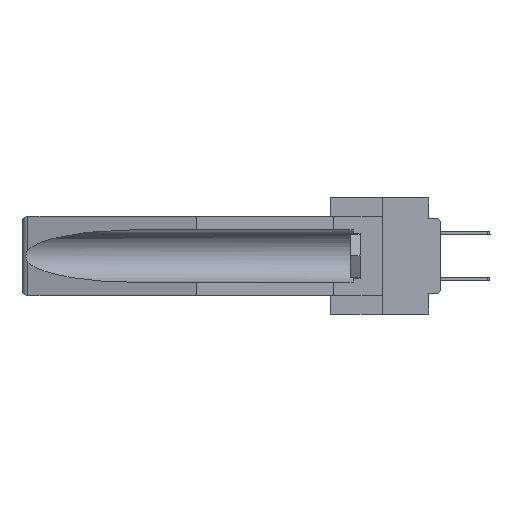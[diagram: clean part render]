
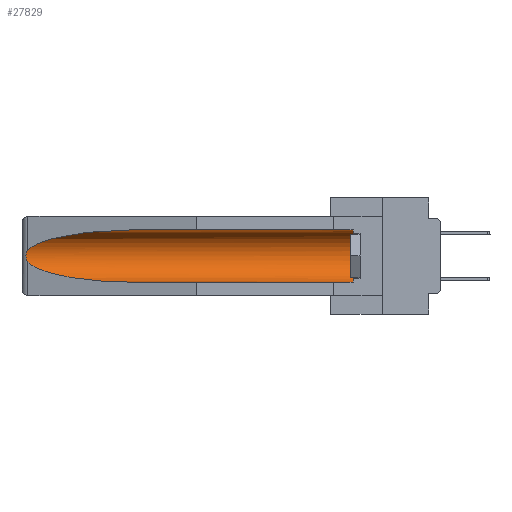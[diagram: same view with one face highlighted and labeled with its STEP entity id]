
A CAD part, left-side view. The second image highlights one B-rep face of the part: STEP entity #27829.
In plain terms, the highlighted cylindrical face has radius 2.857 mm (diameter 5.715 mm), a partial arc.
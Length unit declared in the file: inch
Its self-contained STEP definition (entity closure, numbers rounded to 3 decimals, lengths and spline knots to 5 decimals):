
#566 = VERTEX_POINT ( 'NONE', #17553 ) ;
#653 = CARTESIAN_POINT ( 'NONE',  ( 0.155, 1.07973, -0.059 ) ) ;
#687 = DIRECTION ( 'NONE',  ( 0., 1., 0. ) ) ;
#1659 = LINE ( 'NONE', #16210, #16730 ) ;
#2113 = DIRECTION ( 'NONE',  ( 0., 0., 1. ) ) ;
#2228 = VERTEX_POINT ( 'NONE', #9669 ) ;
#2504 = CARTESIAN_POINT ( 'NONE',  ( 0.155, -0.30754, -0.059 ) ) ;
#3400 = EDGE_LOOP ( 'NONE', ( #4878, #9230, #28040, #16546, #22907, #12775 ) ) ;
#3964 = CARTESIAN_POINT ( 'NONE',  ( 0.2673, 1.5327, -0.16383 ) ) ;
#4175 = CARTESIAN_POINT ( 'NONE',  ( 0.155, 0.126, -0.1715 ) ) ;
#4479 = CARTESIAN_POINT ( 'NONE',  ( 0.155, 1.07973, -0.284 ) ) ;
#4579 = AXIS2_PLACEMENT_3D ( 'NONE', #8742, #15077, #15179 ) ;
#4878 = ORIENTED_EDGE ( 'NONE', *, *, #25182, .T. ) ;
#4927 = FACE_OUTER_BOUND ( 'NONE', #3400, .T. ) ;
#5553 = EDGE_CURVE ( 'NONE', #22213, #27529, #18451, .T. ) ;
#5556 = VERTEX_POINT ( 'NONE', #4479 ) ;
#5742 = CARTESIAN_POINT ( 'NONE',  ( 0.26537, 1.52718, -0.14972 ) ) ;
#6900 = VECTOR ( 'NONE', #22388, 39.37008 ) ;
#7193 =( BOUNDED_CURVE ( )  B_SPLINE_CURVE ( 3, ( #27815, #12310, #20849, #20941 ),
 .UNSPECIFIED., .F., .F. ) 
 B_SPLINE_CURVE_WITH_KNOTS ( ( 4, 4 ),
 ( 0.1948, 1.5708 ),
 .UNSPECIFIED. ) 
 CURVE ( )  GEOMETRIC_REPRESENTATION_ITEM ( )  RATIONAL_B_SPLINE_CURVE ( ( 1., 0.848, 0.848, 1. ) ) 
 REPRESENTATION_ITEM ( '' )  );
#8714 = EDGE_CURVE ( 'NONE', #17061, #2228, #9009, .T. ) ;
#8742 = CARTESIAN_POINT ( 'NONE',  ( 0.155, -0.30754, -0.1715 ) ) ;
#9009 = B_SPLINE_CURVE_WITH_KNOTS ( 'NONE', 3,
 ( #14926, #10539, #17366, #3964, #24130, #10717, #12950, #22350, #15322, #17951 ),
 .UNSPECIFIED., .F., .F.,
 ( 4, 2, 2, 2, 4 ),
 ( 0., 0.00029, 0.00058, 0.00087, 0.00117 ),
 .UNSPECIFIED. ) ;
#9230 = ORIENTED_EDGE ( 'NONE', *, *, #8714, .T. ) ;
#9669 = CARTESIAN_POINT ( 'NONE',  ( 0.26537, 1.52718, -0.19328 ) ) ;
#10539 = CARTESIAN_POINT ( 'NONE',  ( 0.26597, 1.52961, -0.15275 ) ) ;
#10717 = CARTESIAN_POINT ( 'NONE',  ( 0.2675, 1.53308, -0.17534 ) ) ;
#11612 = CARTESIAN_POINT ( 'NONE',  ( 0.21114, 1.30732, -0.059 ) ) ;
#12089 = CARTESIAN_POINT ( 'NONE',  ( 0.25451, 1.48313, -0.09465 ) ) ;
#12310 = CARTESIAN_POINT ( 'NONE',  ( 0.25451, 1.48313, -0.24835 ) ) ;
#12775 = ORIENTED_EDGE ( 'NONE', *, *, #5553, .T. ) ;
#12950 = CARTESIAN_POINT ( 'NONE',  ( 0.2673, 1.53269, -0.17917 ) ) ;
#14926 = CARTESIAN_POINT ( 'NONE',  ( 0.26537, 1.52718, -0.14972 ) ) ;
#15077 = DIRECTION ( 'NONE',  ( 0., 1., 0. ) ) ;
#15137 = CIRCLE ( 'NONE', #19464, 0.1125 ) ;
#15179 = DIRECTION ( 'NONE',  ( 0., 0., 1. ) ) ;
#15322 = CARTESIAN_POINT ( 'NONE',  ( 0.26597, 1.5296, -0.19026 ) ) ;
#15541 = DIRECTION ( 'NONE',  ( 0., -1., 0. ) ) ;
#16210 = CARTESIAN_POINT ( 'NONE',  ( 0.155, -0.30754, -0.284 ) ) ;
#16346 =( BOUNDED_CURVE ( )  B_SPLINE_CURVE ( 3, ( #25039, #11612, #12089, #21002 ),
 .UNSPECIFIED., .F., .T. ) 
 B_SPLINE_CURVE_WITH_KNOTS ( ( 4, 4 ),
 ( 4.71239, 6.08839 ),
 .UNSPECIFIED. ) 
 CURVE ( )  GEOMETRIC_REPRESENTATION_ITEM ( )  RATIONAL_B_SPLINE_CURVE ( ( 1., 0.848, 0.848, 1. ) ) 
 REPRESENTATION_ITEM ( '' )  );
#16498 = CARTESIAN_POINT ( 'NONE',  ( 0.155, 0.126, -0.059 ) ) ;
#16546 = ORIENTED_EDGE ( 'NONE', *, *, #22248, .F. ) ;
#16730 = VECTOR ( 'NONE', #687, 39.37008 ) ;
#17061 = VERTEX_POINT ( 'NONE', #5742 ) ;
#17366 = CARTESIAN_POINT ( 'NONE',  ( 0.26654, 1.53092, -0.15636 ) ) ;
#17553 = CARTESIAN_POINT ( 'NONE',  ( 0.155, 0.126, -0.284 ) ) ;
#17951 = CARTESIAN_POINT ( 'NONE',  ( 0.26537, 1.52718, -0.19328 ) ) ;
#18451 = LINE ( 'NONE', #2504, #6900 ) ;
#19464 = AXIS2_PLACEMENT_3D ( 'NONE', #4175, #15541, #2113 ) ;
#20021 = EDGE_CURVE ( 'NONE', #566, #22213, #15137, .T. ) ;
#20849 = CARTESIAN_POINT ( 'NONE',  ( 0.21114, 1.30732, -0.284 ) ) ;
#20941 = CARTESIAN_POINT ( 'NONE',  ( 0.155, 1.07973, -0.284 ) ) ;
#21002 = CARTESIAN_POINT ( 'NONE',  ( 0.26537, 1.52718, -0.14972 ) ) ;
#22213 = VERTEX_POINT ( 'NONE', #16498 ) ;
#22248 = EDGE_CURVE ( 'NONE', #566, #5556, #1659, .T. ) ;
#22350 = CARTESIAN_POINT ( 'NONE',  ( 0.26655, 1.53094, -0.18657 ) ) ;
#22388 = DIRECTION ( 'NONE',  ( 0., 1., 0. ) ) ;
#22907 = ORIENTED_EDGE ( 'NONE', *, *, #20021, .T. ) ;
#24130 = CARTESIAN_POINT ( 'NONE',  ( 0.2675, 1.53308, -0.16763 ) ) ;
#24516 = CYLINDRICAL_SURFACE ( 'NONE', #4579, 0.1125 ) ;
#25039 = CARTESIAN_POINT ( 'NONE',  ( 0.155, 1.07973, -0.059 ) ) ;
#25182 = EDGE_CURVE ( 'NONE', #27529, #17061, #16346, .T. ) ;
#25740 = EDGE_CURVE ( 'NONE', #2228, #5556, #7193, .T. ) ;
#27529 = VERTEX_POINT ( 'NONE', #653 ) ;
#27815 = CARTESIAN_POINT ( 'NONE',  ( 0.26537, 1.52718, -0.19328 ) ) ;
#27829 = ADVANCED_FACE ( 'NONE', ( #4927 ), #24516, .F. ) ;
#28040 = ORIENTED_EDGE ( 'NONE', *, *, #25740, .T. ) ;
